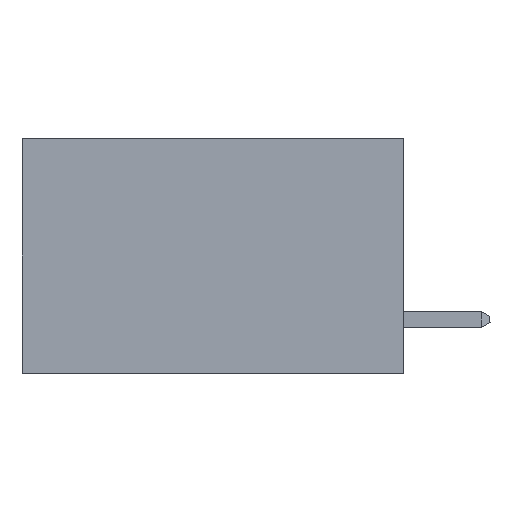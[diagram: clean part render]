
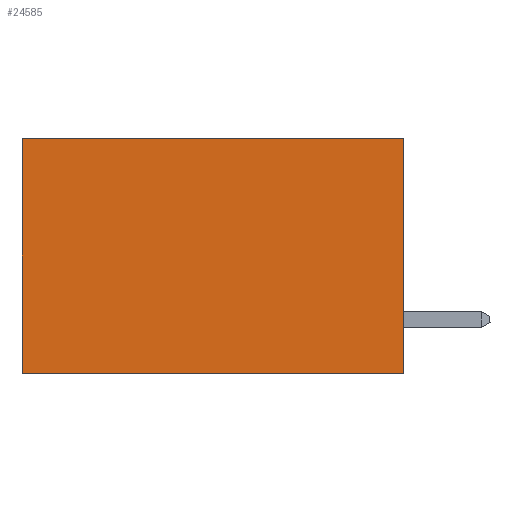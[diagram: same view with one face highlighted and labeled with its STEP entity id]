
A CAD part, left-side view. The second image highlights one B-rep face of the part: STEP entity #24585.
In plain terms, the highlighted planar face has unit normal (-1, 0, 0).
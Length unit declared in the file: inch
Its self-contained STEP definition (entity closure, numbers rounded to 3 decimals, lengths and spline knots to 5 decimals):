
#635 = CARTESIAN_POINT ( 'NONE',  ( 0.2875, 0.6, 0. ) ) ;
#685 = LINE ( 'NONE', #22521, #25227 ) ;
#844 = DIRECTION ( 'NONE',  ( 0., 1., 0. ) ) ;
#1170 = EDGE_CURVE ( 'NONE', #14903, #27120, #26463, .T. ) ;
#1617 = CARTESIAN_POINT ( 'NONE',  ( 0.2875, 0., 0. ) ) ;
#6323 = EDGE_CURVE ( 'NONE', #14903, #26061, #27266, .T. ) ;
#6408 = PLANE ( 'NONE',  #26034 ) ;
#6971 = CARTESIAN_POINT ( 'NONE',  ( 0.2875, 0.6, 0. ) ) ;
#7986 = LINE ( 'NONE', #635, #19445 ) ;
#9267 = DIRECTION ( 'NONE',  ( 0., 0., -1. ) ) ;
#10431 = EDGE_CURVE ( 'NONE', #27120, #27232, #685, .T. ) ;
#12249 = ORIENTED_EDGE ( 'NONE', *, *, #6323, .T. ) ;
#13852 = DIRECTION ( 'NONE',  ( 1., 0., 0. ) ) ;
#14903 = VERTEX_POINT ( 'NONE', #27969 ) ;
#15399 = ORIENTED_EDGE ( 'NONE', *, *, #10431, .F. ) ;
#16855 = DIRECTION ( 'NONE',  ( 0., 0., -1. ) ) ;
#17051 = CARTESIAN_POINT ( 'NONE',  ( 0.2875, 0., 0. ) ) ;
#18501 = ORIENTED_EDGE ( 'NONE', *, *, #1170, .F. ) ;
#19419 = VECTOR ( 'NONE', #16855, 39.37008 ) ;
#19445 = VECTOR ( 'NONE', #28717, 39.37008 ) ;
#19621 = CARTESIAN_POINT ( 'NONE',  ( 0.2875, 0., -0.37 ) ) ;
#21516 = CARTESIAN_POINT ( 'NONE',  ( 0.2875, 0.6, -0.37 ) ) ;
#22286 = FACE_OUTER_BOUND ( 'NONE', #24160, .T. ) ;
#22521 = CARTESIAN_POINT ( 'NONE',  ( 0.2875, 0., -0.37 ) ) ;
#22818 = VECTOR ( 'NONE', #844, 39.37008 ) ;
#24160 = EDGE_LOOP ( 'NONE', ( #29418, #15399, #18501, #12249 ) ) ;
#24585 = ADVANCED_FACE ( 'NONE', ( #22286 ), #6408, .F. ) ;
#25227 = VECTOR ( 'NONE', #29307, 39.37008 ) ;
#26034 = AXIS2_PLACEMENT_3D ( 'NONE', #1617, #13852, #9267 ) ;
#26061 = VERTEX_POINT ( 'NONE', #6971 ) ;
#26453 = EDGE_CURVE ( 'NONE', #26061, #27232, #7986, .T. ) ;
#26463 = LINE ( 'NONE', #17051, #19419 ) ;
#27120 = VERTEX_POINT ( 'NONE', #19621 ) ;
#27232 = VERTEX_POINT ( 'NONE', #21516 ) ;
#27266 = LINE ( 'NONE', #29100, #22818 ) ;
#27969 = CARTESIAN_POINT ( 'NONE',  ( 0.2875, 0., 0. ) ) ;
#28717 = DIRECTION ( 'NONE',  ( 0., 0., -1. ) ) ;
#29100 = CARTESIAN_POINT ( 'NONE',  ( 0.2875, 0., 0. ) ) ;
#29307 = DIRECTION ( 'NONE',  ( 0., 1., 0. ) ) ;
#29418 = ORIENTED_EDGE ( 'NONE', *, *, #26453, .T. ) ;
